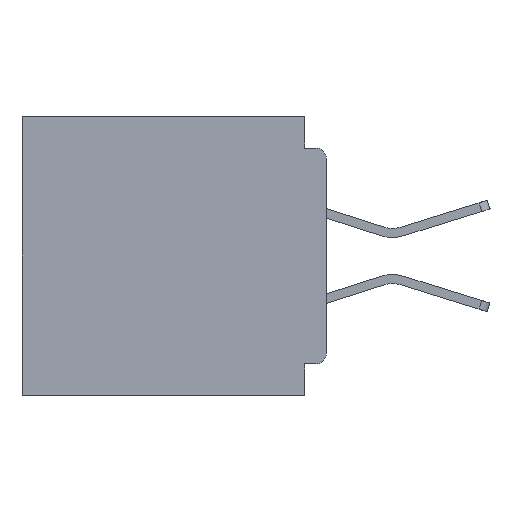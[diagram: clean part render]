
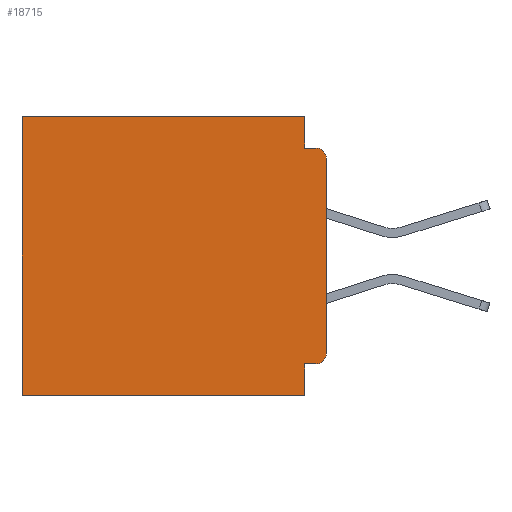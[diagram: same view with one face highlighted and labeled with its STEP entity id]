
A CAD part, left-side view. The second image highlights one B-rep face of the part: STEP entity #18715.
In plain terms, the highlighted planar face has unit normal (-1, 0, 0).
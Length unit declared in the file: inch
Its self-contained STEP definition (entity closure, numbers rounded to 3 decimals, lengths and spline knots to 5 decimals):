
#123 = ORIENTED_EDGE ( 'NONE', *, *, #5646, .T. ) ;
#202 = DIRECTION ( 'NONE',  ( 0., 0., -1. ) ) ;
#449 = PLANE ( 'NONE',  #39214 ) ;
#1279 = ORIENTED_EDGE ( 'NONE', *, *, #34262, .T. ) ;
#1937 = CARTESIAN_POINT ( 'NONE',  ( 0.3, 0.031, -0.355 ) ) ;
#2159 = VECTOR ( 'NONE', #11873, 39.37008 ) ;
#2722 = AXIS2_PLACEMENT_3D ( 'NONE', #35676, #16667, #38788 ) ;
#3174 = VECTOR ( 'NONE', #33797, 39.37008 ) ;
#3391 = CARTESIAN_POINT ( 'NONE',  ( 0.3, 0.031, 0. ) ) ;
#3604 = EDGE_CURVE ( 'NONE', #7860, #24830, #23370, .T. ) ;
#4418 = VERTEX_POINT ( 'NONE', #12258 ) ;
#5646 = EDGE_CURVE ( 'NONE', #16844, #6417, #27151, .T. ) ;
#6411 = VECTOR ( 'NONE', #18979, 39.37008 ) ;
#6417 = VERTEX_POINT ( 'NONE', #17061 ) ;
#6636 = DIRECTION ( 'NONE',  ( 1., 0., 0. ) ) ;
#6774 = VECTOR ( 'NONE', #10445, 39.37008 ) ;
#7860 = VERTEX_POINT ( 'NONE', #20882 ) ;
#8542 = DIRECTION ( 'NONE',  ( 0., 0., -1. ) ) ;
#8637 = CARTESIAN_POINT ( 'NONE',  ( 0.3, 0.031, -0.4 ) ) ;
#9462 = ORIENTED_EDGE ( 'NONE', *, *, #27798, .T. ) ;
#10134 = CARTESIAN_POINT ( 'NONE',  ( 0.3, 0.031, 0. ) ) ;
#10283 = VERTEX_POINT ( 'NONE', #28290 ) ;
#10309 = EDGE_CURVE ( 'NONE', #16844, #21369, #30760, .T. ) ;
#10445 = DIRECTION ( 'NONE',  ( 0., 1., 0. ) ) ;
#10718 = ORIENTED_EDGE ( 'NONE', *, *, #18851, .F. ) ;
#10854 = ORIENTED_EDGE ( 'NONE', *, *, #38330, .F. ) ;
#11288 = CARTESIAN_POINT ( 'NONE',  ( 0.3, 0.437, -0.4 ) ) ;
#11300 = VECTOR ( 'NONE', #202, 39.37008 ) ;
#11593 = CARTESIAN_POINT ( 'NONE',  ( 0.3, 0., -0.045 ) ) ;
#11873 = DIRECTION ( 'NONE',  ( 0., 0., -1. ) ) ;
#12074 = FACE_OUTER_BOUND ( 'NONE', #35622, .T. ) ;
#12258 = CARTESIAN_POINT ( 'NONE',  ( 0.3, 0.031, -0.4 ) ) ;
#13041 = ORIENTED_EDGE ( 'NONE', *, *, #26079, .F. ) ;
#13395 = LINE ( 'NONE', #23753, #35729 ) ;
#13813 = CARTESIAN_POINT ( 'NONE',  ( 0.3, 0., -0.06 ) ) ;
#13895 = VECTOR ( 'NONE', #8542, 39.37008 ) ;
#14078 = EDGE_CURVE ( 'NONE', #10283, #6417, #26520, .T. ) ;
#15184 = ORIENTED_EDGE ( 'NONE', *, *, #10309, .F. ) ;
#15471 = EDGE_CURVE ( 'NONE', #34223, #10283, #38551, .T. ) ;
#15507 = ORIENTED_EDGE ( 'NONE', *, *, #15471, .F. ) ;
#15558 = LINE ( 'NONE', #38881, #31417 ) ;
#16233 = CARTESIAN_POINT ( 'NONE',  ( 0.3, 0., -0.4 ) ) ;
#16384 = AXIS2_PLACEMENT_3D ( 'NONE', #19855, #19845, #19797 ) ;
#16667 = DIRECTION ( 'NONE',  ( -1., 0., 0. ) ) ;
#16844 = VERTEX_POINT ( 'NONE', #13813 ) ;
#17061 = CARTESIAN_POINT ( 'NONE',  ( 0.3, 0.015, -0.045 ) ) ;
#18113 = CARTESIAN_POINT ( 'NONE',  ( 0.3, 0., -0.34 ) ) ;
#18138 = CARTESIAN_POINT ( 'NONE',  ( 0.3, 0.015, -0.355 ) ) ;
#18620 = ORIENTED_EDGE ( 'NONE', *, *, #14078, .F. ) ;
#18715 = ADVANCED_FACE ( 'NONE', ( #12074 ), #449, .F. ) ;
#18851 = EDGE_CURVE ( 'NONE', #4418, #24830, #15558, .T. ) ;
#18979 = DIRECTION ( 'NONE',  ( 0., 0., -1. ) ) ;
#19797 = DIRECTION ( 'NONE',  ( 0., 0., -1. ) ) ;
#19845 = DIRECTION ( 'NONE',  ( -1., 0., 0. ) ) ;
#19855 = CARTESIAN_POINT ( 'NONE',  ( 0.3, 0.015, -0.06 ) ) ;
#19958 = DIRECTION ( 'NONE',  ( 0., 1., 0. ) ) ;
#20882 = CARTESIAN_POINT ( 'NONE',  ( 0.3, 0.437, 0. ) ) ;
#21369 = VERTEX_POINT ( 'NONE', #18113 ) ;
#22641 = DIRECTION ( 'NONE',  ( 0., 0., -1. ) ) ;
#23370 = LINE ( 'NONE', #11288, #13895 ) ;
#23753 = CARTESIAN_POINT ( 'NONE',  ( 0.3, 0., -0.355 ) ) ;
#23820 = CIRCLE ( 'NONE', #2722, 0.015 ) ;
#24830 = VERTEX_POINT ( 'NONE', #27162 ) ;
#26079 = EDGE_CURVE ( 'NONE', #28647, #27335, #13395, .T. ) ;
#26520 = LINE ( 'NONE', #11593, #3174 ) ;
#27151 = CIRCLE ( 'NONE', #16384, 0.015 ) ;
#27162 = CARTESIAN_POINT ( 'NONE',  ( 0.3, 0.437, -0.4 ) ) ;
#27335 = VERTEX_POINT ( 'NONE', #1937 ) ;
#27798 = EDGE_CURVE ( 'NONE', #34223, #7860, #32095, .T. ) ;
#28290 = CARTESIAN_POINT ( 'NONE',  ( 0.3, 0.031, -0.045 ) ) ;
#28422 = LINE ( 'NONE', #8637, #2159 ) ;
#28647 = VERTEX_POINT ( 'NONE', #18138 ) ;
#30760 = LINE ( 'NONE', #37935, #6411 ) ;
#31417 = VECTOR ( 'NONE', #19958, 39.37008 ) ;
#32095 = LINE ( 'NONE', #32630, #6774 ) ;
#32630 = CARTESIAN_POINT ( 'NONE',  ( 0.3, 0., 0. ) ) ;
#33797 = DIRECTION ( 'NONE',  ( 0., -1., 0. ) ) ;
#34117 = ORIENTED_EDGE ( 'NONE', *, *, #3604, .T. ) ;
#34223 = VERTEX_POINT ( 'NONE', #10134 ) ;
#34262 = EDGE_CURVE ( 'NONE', #28647, #21369, #23820, .T. ) ;
#35622 = EDGE_LOOP ( 'NONE', ( #15184, #123, #18620, #15507, #9462, #34117, #10718, #10854, #13041, #1279 ) ) ;
#35676 = CARTESIAN_POINT ( 'NONE',  ( 0.3, 0.015, -0.34 ) ) ;
#35729 = VECTOR ( 'NONE', #36305, 39.37008 ) ;
#36305 = DIRECTION ( 'NONE',  ( 0., 1., 0. ) ) ;
#37935 = CARTESIAN_POINT ( 'NONE',  ( 0.3, 0., -0.4 ) ) ;
#38330 = EDGE_CURVE ( 'NONE', #27335, #4418, #28422, .T. ) ;
#38551 = LINE ( 'NONE', #3391, #11300 ) ;
#38788 = DIRECTION ( 'NONE',  ( 0., 0., -1. ) ) ;
#38881 = CARTESIAN_POINT ( 'NONE',  ( 0.3, 0., -0.4 ) ) ;
#39214 = AXIS2_PLACEMENT_3D ( 'NONE', #16233, #6636, #22641 ) ;
